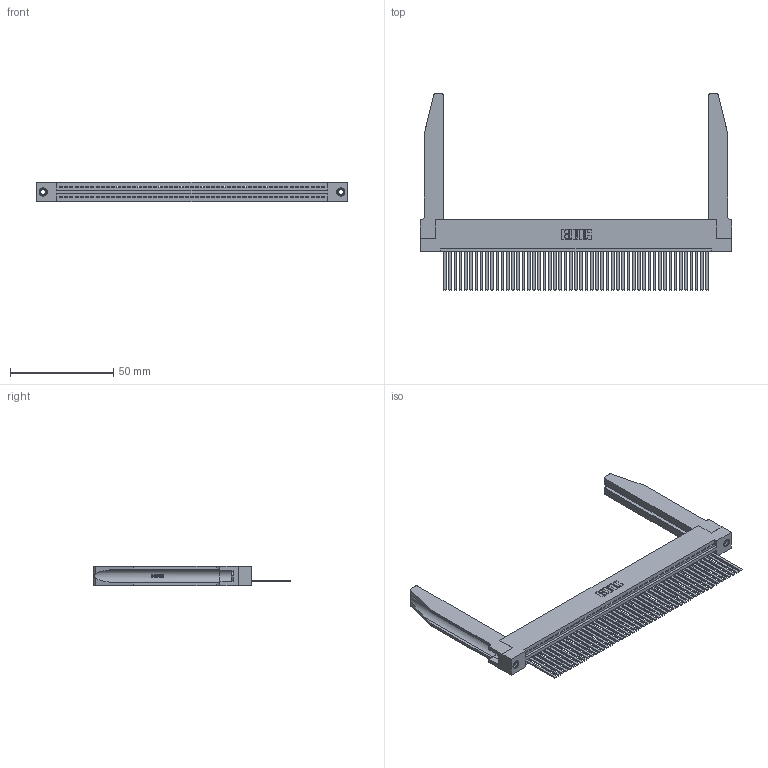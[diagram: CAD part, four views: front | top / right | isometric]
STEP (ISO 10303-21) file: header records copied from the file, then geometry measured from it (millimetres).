
FILE_DESCRIPTION (( 'STEP AP203' ), '1' );
FILE_NAME ('395-051-544-178.STEP', '2019-10-23T11:07:36', ( '' ), ( '' ), 'SwSTEP 2.0', 'SolidWorks 2016', '' );
FILE_SCHEMA (( 'CONFIG_CONTROL_DESIGN' ));
Length unit declared in the file: inch
Products named in the file (5): 345-250-001_345-250-001-102; 395-051-544-178; 345-220-078_345-220-078; 345-292-001_345-293-144; 345 Part_Flush Mounting Lugs - 0.156 Dia-TH
Assembly tree (56 placements, depth 2):
  395-051-544-178
    345 Part_Flush Mounting Lugs - 0.156 Dia-TH
    345-292-001_345-293-144  x51
    345-250-001_345-250-001-102  x2
    345-220-078_345-220-078  x2
Bounding box: 150.77 x 94.92 x 9.4 mm (x, y, z)
Volume: 22755.6 mm3; surface area: 28654.9 mm2
Topology: 56 solids, 56 shells, 3012 faces, 9007 edges, 5926 vertices
Faces by surface type: plane 2058, cylinder 902, bspline 36, cone 12, torus 4
Entity records: 41728 total; most frequent: CARTESIAN_POINT 8124, ORIENTED_EDGE 7006, DIRECTION 6087, EDGE_CURVE 3503, LINE 3077, VECTOR 3077, VERTEX_POINT 2328, AXIS2_PLACEMENT_3D 1505
